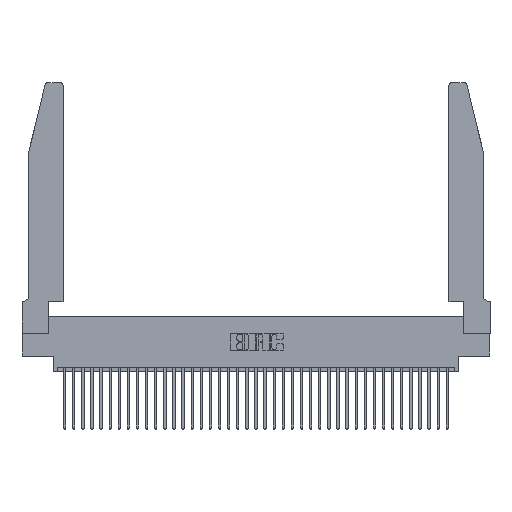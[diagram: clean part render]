
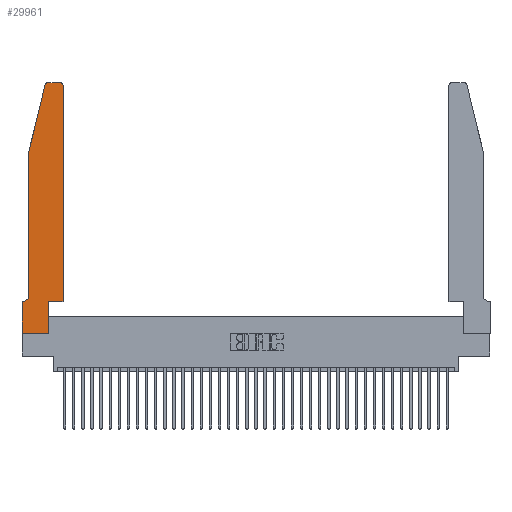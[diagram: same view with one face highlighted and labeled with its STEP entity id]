
A CAD part, top view. The second image highlights one B-rep face of the part: STEP entity #29961.
In plain terms, the highlighted planar face has unit normal (0, 0, 1).
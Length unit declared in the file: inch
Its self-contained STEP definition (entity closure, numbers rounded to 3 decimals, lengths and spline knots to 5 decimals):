
#1424 = DIRECTION ( 'NONE',  ( 0., 1., 0. ) ) ;
#2335 = VERTEX_POINT ( 'NONE', #15672 ) ;
#2531 = LINE ( 'NONE', #10228, #26489 ) ;
#2607 = VERTEX_POINT ( 'NONE', #14229 ) ;
#2758 = VERTEX_POINT ( 'NONE', #35393 ) ;
#2891 = CIRCLE ( 'NONE', #21998, 0.03 ) ;
#3091 = DIRECTION ( 'NONE',  ( 0., 0., 1. ) ) ;
#3807 = EDGE_CURVE ( 'NONE', #11602, #5596, #9452, .T. ) ;
#3817 = ORIENTED_EDGE ( 'NONE', *, *, #3807, .T. ) ;
#4314 = ORIENTED_EDGE ( 'NONE', *, *, #18455, .T. ) ;
#5103 = ORIENTED_EDGE ( 'NONE', *, *, #32735, .T. ) ;
#5184 = VECTOR ( 'NONE', #29842, 39.37008 ) ;
#5334 = ORIENTED_EDGE ( 'NONE', *, *, #21483, .T. ) ;
#5496 = VECTOR ( 'NONE', #23721, 39.37008 ) ;
#5596 = VERTEX_POINT ( 'NONE', #14808 ) ;
#7190 = VECTOR ( 'NONE', #37671, 39.37008 ) ;
#7356 = ORIENTED_EDGE ( 'NONE', *, *, #10792, .T. ) ;
#7458 = CARTESIAN_POINT ( 'NONE',  ( 0.2865, 0.35, 0.37 ) ) ;
#8488 = VECTOR ( 'NONE', #23455, 39.37008 ) ;
#8602 = ORIENTED_EDGE ( 'NONE', *, *, #25763, .T. ) ;
#8709 = CARTESIAN_POINT ( 'NONE',  ( 0.0755, 2., 0.37 ) ) ;
#8940 = LINE ( 'NONE', #37902, #23896 ) ;
#9452 = LINE ( 'NONE', #26408, #8488 ) ;
#9654 = CARTESIAN_POINT ( 'NONE',  ( 0.2605, 2.75, 0.37 ) ) ;
#10064 = AXIS2_PLACEMENT_3D ( 'NONE', #11132, #31768, #14176 ) ;
#10082 = ORIENTED_EDGE ( 'NONE', *, *, #35749, .T. ) ;
#10228 = CARTESIAN_POINT ( 'NONE',  ( 0.0755, 2., 0.37 ) ) ;
#10681 = EDGE_CURVE ( 'NONE', #38026, #31447, #2891, .T. ) ;
#10700 = ORIENTED_EDGE ( 'NONE', *, *, #28567, .T. ) ;
#10792 = EDGE_CURVE ( 'NONE', #31447, #32264, #29096, .T. ) ;
#11132 = CARTESIAN_POINT ( 'NONE',  ( 0.284, 2.72, 0.37 ) ) ;
#11602 = VERTEX_POINT ( 'NONE', #33499 ) ;
#11711 = CARTESIAN_POINT ( 'NONE',  ( 0., 0.35, 0.37 ) ) ;
#11732 = EDGE_CURVE ( 'NONE', #2335, #38026, #13881, .T. ) ;
#12109 = CARTESIAN_POINT ( 'NONE',  ( 0.25487, 2.72718, 0.37 ) ) ;
#12989 = CARTESIAN_POINT ( 'NONE',  ( 0.284, 2.75, 0.37 ) ) ;
#13223 = VECTOR ( 'NONE', #18728, 39.37008 ) ;
#13628 = LINE ( 'NONE', #8709, #5496 ) ;
#13881 = LINE ( 'NONE', #37065, #28635 ) ;
#13964 = DIRECTION ( 'NONE',  ( 0., 0., -1. ) ) ;
#14176 = DIRECTION ( 'NONE',  ( 1., 0., 0. ) ) ;
#14229 = CARTESIAN_POINT ( 'NONE',  ( 0.0755, 0.42, 0.37 ) ) ;
#14347 = ORIENTED_EDGE ( 'NONE', *, *, #22665, .T. ) ;
#14735 = DIRECTION ( 'NONE',  ( 0., 0., 1. ) ) ;
#14808 = CARTESIAN_POINT ( 'NONE',  ( 0., 0., 0.37 ) ) ;
#15575 = CARTESIAN_POINT ( 'NONE',  ( 0.4505, 2.72, 0.37 ) ) ;
#15672 = CARTESIAN_POINT ( 'NONE',  ( 0.4505, 0.35, 0.37 ) ) ;
#15767 = CARTESIAN_POINT ( 'NONE',  ( 0.2865, 0.35, 0.37 ) ) ;
#16162 = DIRECTION ( 'NONE',  ( 0., -1., 0. ) ) ;
#17196 = CARTESIAN_POINT ( 'NONE',  ( 0., 0., 0.37 ) ) ;
#17438 = DIRECTION ( 'NONE',  ( -1., 0., 0. ) ) ;
#18270 = CIRCLE ( 'NONE', #10064, 0.03 ) ;
#18307 = ORIENTED_EDGE ( 'NONE', *, *, #11732, .T. ) ;
#18455 = EDGE_CURVE ( 'NONE', #2758, #11602, #8940, .T. ) ;
#18688 = DIRECTION ( 'NONE',  ( -1., 0., 0. ) ) ;
#18728 = DIRECTION ( 'NONE',  ( 0., 1., 0. ) ) ;
#19082 = ORIENTED_EDGE ( 'NONE', *, *, #34719, .T. ) ;
#20546 = CIRCLE ( 'NONE', #23227, 0.07 ) ;
#21178 = CARTESIAN_POINT ( 'NONE',  ( 0.4205, 2.72, 0.37 ) ) ;
#21298 = VECTOR ( 'NONE', #18688, 39.37008 ) ;
#21483 = EDGE_CURVE ( 'NONE', #37259, #27417, #37538, .T. ) ;
#21629 = ORIENTED_EDGE ( 'NONE', *, *, #10681, .T. ) ;
#21998 = AXIS2_PLACEMENT_3D ( 'NONE', #21178, #3091, #24132 ) ;
#22665 = EDGE_CURVE ( 'NONE', #2607, #2758, #20546, .T. ) ;
#23128 = LINE ( 'NONE', #17196, #7190 ) ;
#23227 = AXIS2_PLACEMENT_3D ( 'NONE', #31566, #13964, #34480 ) ;
#23388 = VERTEX_POINT ( 'NONE', #32917 ) ;
#23455 = DIRECTION ( 'NONE',  ( 0., -1., 0. ) ) ;
#23721 = DIRECTION ( 'NONE',  ( -0.239, -0.971, 0. ) ) ;
#23896 = VECTOR ( 'NONE', #17438, 39.37008 ) ;
#24132 = DIRECTION ( 'NONE',  ( 1., 0., 0. ) ) ;
#24703 = FACE_OUTER_BOUND ( 'NONE', #37387, .T. ) ;
#25763 = EDGE_CURVE ( 'NONE', #5596, #37259, #23128, .T. ) ;
#26408 = CARTESIAN_POINT ( 'NONE',  ( 0., 0., 0.37 ) ) ;
#26489 = VECTOR ( 'NONE', #16162, 39.37008 ) ;
#27029 = AXIS2_PLACEMENT_3D ( 'NONE', #11711, #14735, #35268 ) ;
#27417 = VERTEX_POINT ( 'NONE', #7458 ) ;
#28567 = EDGE_CURVE ( 'NONE', #32264, #33363, #18270, .T. ) ;
#28635 = VECTOR ( 'NONE', #1424, 39.37008 ) ;
#29096 = LINE ( 'NONE', #9654, #21298 ) ;
#29842 = DIRECTION ( 'NONE',  ( 1., 0., 0. ) ) ;
#29914 = LINE ( 'NONE', #32759, #5184 ) ;
#29961 = ADVANCED_FACE ( 'NONE', ( #24703 ), #32332, .T. ) ;
#31447 = VERTEX_POINT ( 'NONE', #32851 ) ;
#31566 = CARTESIAN_POINT ( 'NONE',  ( 0.0055, 0.42, 0.37 ) ) ;
#31768 = DIRECTION ( 'NONE',  ( 0., 0., 1. ) ) ;
#32264 = VERTEX_POINT ( 'NONE', #12989 ) ;
#32332 = PLANE ( 'NONE',  #27029 ) ;
#32735 = EDGE_CURVE ( 'NONE', #27417, #2335, #29914, .T. ) ;
#32759 = CARTESIAN_POINT ( 'NONE',  ( 0.4505, 0.35, 0.37 ) ) ;
#32851 = CARTESIAN_POINT ( 'NONE',  ( 0.4205, 2.75, 0.37 ) ) ;
#32917 = CARTESIAN_POINT ( 'NONE',  ( 0.0755, 2., 0.37 ) ) ;
#33363 = VERTEX_POINT ( 'NONE', #12109 ) ;
#33499 = CARTESIAN_POINT ( 'NONE',  ( 0., 0.35, 0.37 ) ) ;
#34480 = DIRECTION ( 'NONE',  ( -1., 0., 0. ) ) ;
#34719 = EDGE_CURVE ( 'NONE', #33363, #23388, #13628, .T. ) ;
#35268 = DIRECTION ( 'NONE',  ( 1., 0., 0. ) ) ;
#35393 = CARTESIAN_POINT ( 'NONE',  ( 0.0055, 0.35, 0.37 ) ) ;
#35749 = EDGE_CURVE ( 'NONE', #23388, #2607, #2531, .T. ) ;
#37065 = CARTESIAN_POINT ( 'NONE',  ( 0.4505, 0.35, 0.37 ) ) ;
#37259 = VERTEX_POINT ( 'NONE', #37659 ) ;
#37387 = EDGE_LOOP ( 'NONE', ( #7356, #10700, #19082, #10082, #14347, #4314, #3817, #8602, #5334, #5103, #18307, #21629 ) ) ;
#37538 = LINE ( 'NONE', #15767, #13223 ) ;
#37659 = CARTESIAN_POINT ( 'NONE',  ( 0.2865, 0., 0.37 ) ) ;
#37671 = DIRECTION ( 'NONE',  ( 1., 0., 0. ) ) ;
#37902 = CARTESIAN_POINT ( 'NONE',  ( 0.0755, 0.35, 0.37 ) ) ;
#38026 = VERTEX_POINT ( 'NONE', #15575 ) ;
